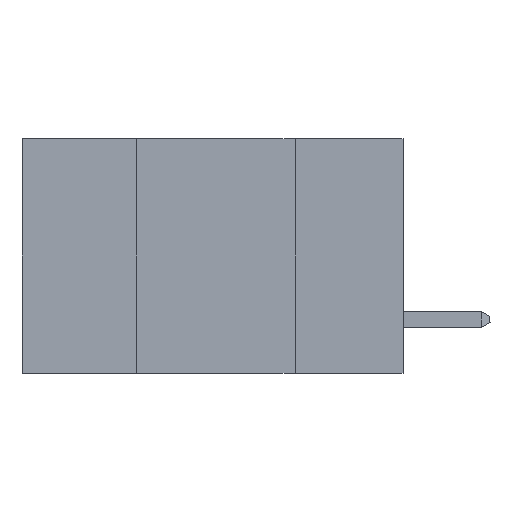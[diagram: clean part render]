
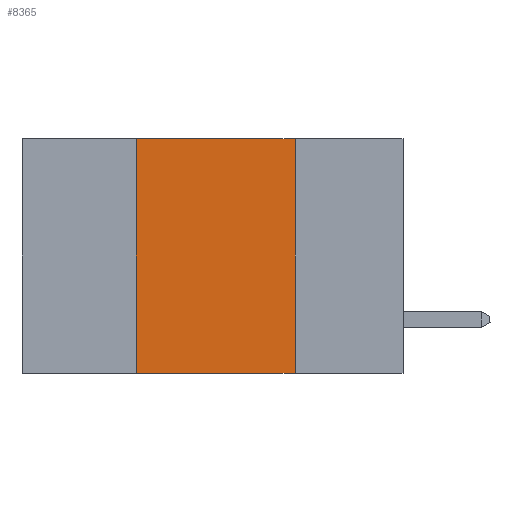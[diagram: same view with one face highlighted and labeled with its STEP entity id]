
A CAD part, left-side view. The second image highlights one B-rep face of the part: STEP entity #8365.
In plain terms, the highlighted planar face has unit normal (-1, 0, 0).
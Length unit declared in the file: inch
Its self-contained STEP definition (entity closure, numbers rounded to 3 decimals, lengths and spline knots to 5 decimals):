
#562 = EDGE_CURVE ( 'NONE', #2328, #10320, #11669, .T. ) ;
#655 = CARTESIAN_POINT ( 'NONE',  ( 0., 0.17, 0. ) ) ;
#826 = AXIS2_PLACEMENT_3D ( 'NONE', #7954, #14535, #14424 ) ;
#1162 = VECTOR ( 'NONE', #13117, 39.37008 ) ;
#1617 = EDGE_CURVE ( 'NONE', #10320, #15915, #4311, .T. ) ;
#2328 = VERTEX_POINT ( 'NONE', #7248 ) ;
#2517 = CARTESIAN_POINT ( 'NONE',  ( 0., 0.17, -0.37 ) ) ;
#2724 = VECTOR ( 'NONE', #7172, 39.37008 ) ;
#3588 = EDGE_LOOP ( 'NONE', ( #9006, #11520, #15375, #8865 ) ) ;
#3910 = PLANE ( 'NONE',  #826 ) ;
#4311 = LINE ( 'NONE', #5430, #14730 ) ;
#4796 = LINE ( 'NONE', #655, #2724 ) ;
#5430 = CARTESIAN_POINT ( 'NONE',  ( 0., 0.6, 0. ) ) ;
#5905 = LINE ( 'NONE', #13340, #1162 ) ;
#7172 = DIRECTION ( 'NONE',  ( 0., 0., -1. ) ) ;
#7248 = CARTESIAN_POINT ( 'NONE',  ( 0., 0.42, -0.37 ) ) ;
#7599 = EDGE_CURVE ( 'NONE', #15915, #10322, #4796, .T. ) ;
#7954 = CARTESIAN_POINT ( 'NONE',  ( 0., 0.6, 0. ) ) ;
#8023 = CARTESIAN_POINT ( 'NONE',  ( 0., 0.42, 0. ) ) ;
#8176 = DIRECTION ( 'NONE',  ( 0., -1., 0. ) ) ;
#8263 = VECTOR ( 'NONE', #15752, 39.37008 ) ;
#8365 = ADVANCED_FACE ( 'NONE', ( #13949 ), #3910, .F. ) ;
#8865 = ORIENTED_EDGE ( 'NONE', *, *, #16237, .T. ) ;
#9006 = ORIENTED_EDGE ( 'NONE', *, *, #7599, .F. ) ;
#9651 = CARTESIAN_POINT ( 'NONE',  ( 0., 0.17, 0. ) ) ;
#10320 = VERTEX_POINT ( 'NONE', #11424 ) ;
#10322 = VERTEX_POINT ( 'NONE', #2517 ) ;
#11424 = CARTESIAN_POINT ( 'NONE',  ( 0., 0.42, 0. ) ) ;
#11520 = ORIENTED_EDGE ( 'NONE', *, *, #1617, .F. ) ;
#11669 = LINE ( 'NONE', #8023, #8263 ) ;
#13117 = DIRECTION ( 'NONE',  ( 0., -1., 0. ) ) ;
#13340 = CARTESIAN_POINT ( 'NONE',  ( 0., 0.6, -0.37 ) ) ;
#13949 = FACE_OUTER_BOUND ( 'NONE', #3588, .T. ) ;
#14424 = DIRECTION ( 'NONE',  ( 0., 0., -1. ) ) ;
#14535 = DIRECTION ( 'NONE',  ( 1., 0., 0. ) ) ;
#14730 = VECTOR ( 'NONE', #8176, 39.37008 ) ;
#15375 = ORIENTED_EDGE ( 'NONE', *, *, #562, .F. ) ;
#15752 = DIRECTION ( 'NONE',  ( 0., 0., 1. ) ) ;
#15915 = VERTEX_POINT ( 'NONE', #9651 ) ;
#16237 = EDGE_CURVE ( 'NONE', #2328, #10322, #5905, .T. ) ;
